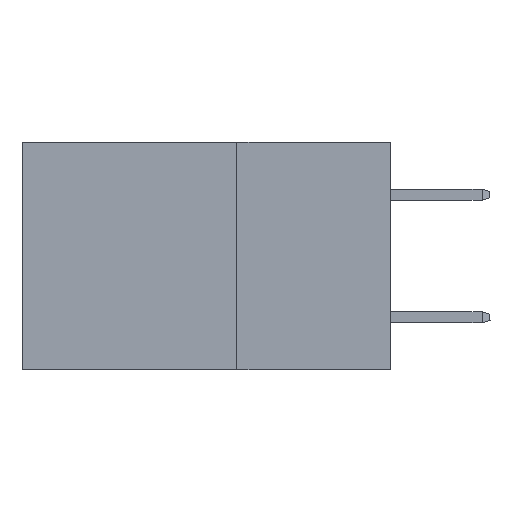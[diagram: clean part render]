
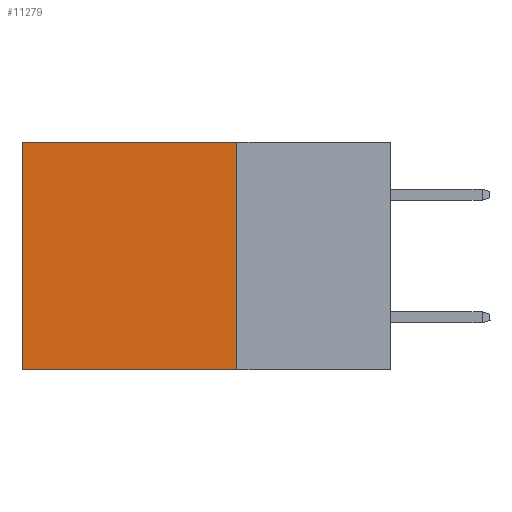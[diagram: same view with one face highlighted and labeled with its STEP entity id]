
A CAD part, left-side view. The second image highlights one B-rep face of the part: STEP entity #11279.
In plain terms, the highlighted planar face has unit normal (-1, 0, 0).
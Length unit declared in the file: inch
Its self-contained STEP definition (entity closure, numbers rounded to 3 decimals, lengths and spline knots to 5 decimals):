
#157 = LINE ( 'NONE', #8391, #5846 ) ;
#1363 = CARTESIAN_POINT ( 'NONE',  ( 0.2875, 0.6, 0. ) ) ;
#1899 = CARTESIAN_POINT ( 'NONE',  ( 0.2875, 0.25, -0.37 ) ) ;
#2095 = EDGE_CURVE ( 'NONE', #9186, #17894, #3461, .T. ) ;
#3185 = ORIENTED_EDGE ( 'NONE', *, *, #22647, .F. ) ;
#3461 = LINE ( 'NONE', #21088, #9586 ) ;
#3932 = CARTESIAN_POINT ( 'NONE',  ( 0.2875, 0.25, 0. ) ) ;
#5824 = AXIS2_PLACEMENT_3D ( 'NONE', #3932, #20613, #12335 ) ;
#5846 = VECTOR ( 'NONE', #6580, 39.37008 ) ;
#5900 = FACE_OUTER_BOUND ( 'NONE', #7008, .T. ) ;
#6580 = DIRECTION ( 'NONE',  ( 0., 0., -1. ) ) ;
#7008 = EDGE_LOOP ( 'NONE', ( #16771, #3185, #9638, #21884 ) ) ;
#8391 = CARTESIAN_POINT ( 'NONE',  ( 0.2875, 0.25, 0. ) ) ;
#9186 = VERTEX_POINT ( 'NONE', #1363 ) ;
#9586 = VECTOR ( 'NONE', #10434, 39.37008 ) ;
#9604 = VECTOR ( 'NONE', #22197, 39.37008 ) ;
#9638 = ORIENTED_EDGE ( 'NONE', *, *, #11385, .F. ) ;
#10434 = DIRECTION ( 'NONE',  ( 0., 0., -1. ) ) ;
#11128 = CARTESIAN_POINT ( 'NONE',  ( 0.2875, 0.25, 0. ) ) ;
#11279 = ADVANCED_FACE ( 'NONE', ( #5900 ), #18354, .F. ) ;
#11385 = EDGE_CURVE ( 'NONE', #20201, #14493, #157, .T. ) ;
#12335 = DIRECTION ( 'NONE',  ( 0., 0., -1. ) ) ;
#13687 = CARTESIAN_POINT ( 'NONE',  ( 0.2875, 0.25, 0. ) ) ;
#14493 = VERTEX_POINT ( 'NONE', #1899 ) ;
#15334 = LINE ( 'NONE', #11128, #9604 ) ;
#15460 = EDGE_CURVE ( 'NONE', #20201, #9186, #15334, .T. ) ;
#16063 = CARTESIAN_POINT ( 'NONE',  ( 0.2875, 0.25, -0.37 ) ) ;
#16483 = DIRECTION ( 'NONE',  ( 0., 1., 0. ) ) ;
#16771 = ORIENTED_EDGE ( 'NONE', *, *, #2095, .T. ) ;
#17522 = CARTESIAN_POINT ( 'NONE',  ( 0.2875, 0.6, -0.37 ) ) ;
#17894 = VERTEX_POINT ( 'NONE', #17522 ) ;
#18354 = PLANE ( 'NONE',  #5824 ) ;
#18757 = VECTOR ( 'NONE', #16483, 39.37008 ) ;
#20201 = VERTEX_POINT ( 'NONE', #13687 ) ;
#20613 = DIRECTION ( 'NONE',  ( 1., 0., 0. ) ) ;
#21088 = CARTESIAN_POINT ( 'NONE',  ( 0.2875, 0.6, 0. ) ) ;
#21884 = ORIENTED_EDGE ( 'NONE', *, *, #15460, .T. ) ;
#22197 = DIRECTION ( 'NONE',  ( 0., 1., 0. ) ) ;
#22379 = LINE ( 'NONE', #16063, #18757 ) ;
#22647 = EDGE_CURVE ( 'NONE', #14493, #17894, #22379, .T. ) ;
